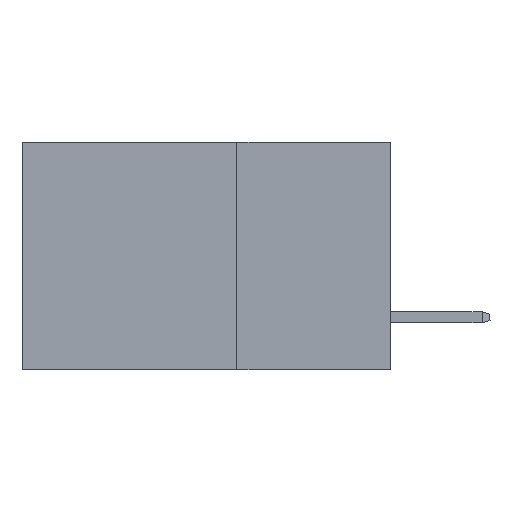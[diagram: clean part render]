
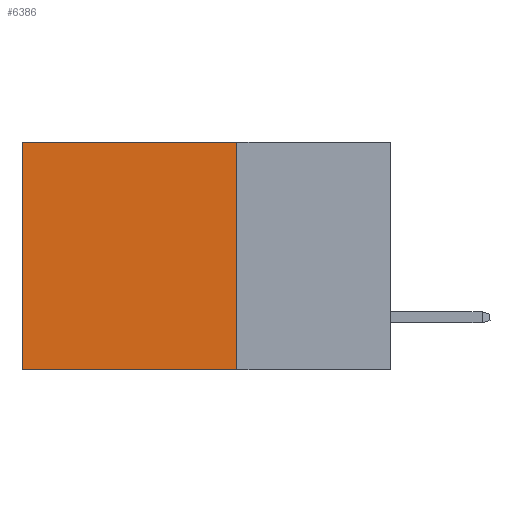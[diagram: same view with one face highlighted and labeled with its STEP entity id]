
A CAD part, left-side view. The second image highlights one B-rep face of the part: STEP entity #6386.
In plain terms, the highlighted planar face has unit normal (-1, 0, 0).
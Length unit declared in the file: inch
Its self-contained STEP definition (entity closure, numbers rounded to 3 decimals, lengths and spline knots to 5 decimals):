
#364 = CARTESIAN_POINT ( 'NONE',  ( 0.2875, 0.6, -0.37 ) ) ;
#1984 = CARTESIAN_POINT ( 'NONE',  ( 0.2875, 0.25, -0.37 ) ) ;
#2089 = DIRECTION ( 'NONE',  ( 0., 1., 0. ) ) ;
#3201 = EDGE_CURVE ( 'NONE', #13174, #11558, #13690, .T. ) ;
#3817 = ORIENTED_EDGE ( 'NONE', *, *, #20676, .F. ) ;
#4170 = ORIENTED_EDGE ( 'NONE', *, *, #3201, .T. ) ;
#4870 = CARTESIAN_POINT ( 'NONE',  ( 0.2875, 0.6, 0. ) ) ;
#5014 = VERTEX_POINT ( 'NONE', #11487 ) ;
#5525 = EDGE_CURVE ( 'NONE', #5014, #10387, #21760, .T. ) ;
#6386 = ADVANCED_FACE ( 'NONE', ( #8732 ), #9446, .F. ) ;
#7479 = CARTESIAN_POINT ( 'NONE',  ( 0.2875, 0.25, 0. ) ) ;
#8732 = FACE_OUTER_BOUND ( 'NONE', #17530, .T. ) ;
#9446 = PLANE ( 'NONE',  #27408 ) ;
#9730 = CARTESIAN_POINT ( 'NONE',  ( 0.2875, 0.25, 0. ) ) ;
#10387 = VERTEX_POINT ( 'NONE', #364 ) ;
#10723 = CARTESIAN_POINT ( 'NONE',  ( 0.2875, 0.6, 0. ) ) ;
#10885 = VECTOR ( 'NONE', #28116, 39.37008 ) ;
#11487 = CARTESIAN_POINT ( 'NONE',  ( 0.2875, 0.25, -0.37 ) ) ;
#11558 = VERTEX_POINT ( 'NONE', #4870 ) ;
#13174 = VERTEX_POINT ( 'NONE', #24351 ) ;
#13477 = LINE ( 'NONE', #9730, #25055 ) ;
#13690 = LINE ( 'NONE', #7479, #19503 ) ;
#13816 = DIRECTION ( 'NONE',  ( 0., 0., -1. ) ) ;
#14179 = EDGE_CURVE ( 'NONE', #11558, #10387, #28245, .T. ) ;
#17530 = EDGE_LOOP ( 'NONE', ( #19243, #17594, #3817, #4170 ) ) ;
#17594 = ORIENTED_EDGE ( 'NONE', *, *, #5525, .F. ) ;
#18402 = DIRECTION ( 'NONE',  ( 0., 0., -1. ) ) ;
#19243 = ORIENTED_EDGE ( 'NONE', *, *, #14179, .T. ) ;
#19503 = VECTOR ( 'NONE', #2089, 39.37008 ) ;
#20676 = EDGE_CURVE ( 'NONE', #13174, #5014, #13477, .T. ) ;
#21760 = LINE ( 'NONE', #1984, #26078 ) ;
#24351 = CARTESIAN_POINT ( 'NONE',  ( 0.2875, 0.25, 0. ) ) ;
#24649 = CARTESIAN_POINT ( 'NONE',  ( 0.2875, 0.25, 0. ) ) ;
#25055 = VECTOR ( 'NONE', #18402, 39.37008 ) ;
#26078 = VECTOR ( 'NONE', #28215, 39.37008 ) ;
#26808 = DIRECTION ( 'NONE',  ( 1., 0., 0. ) ) ;
#27408 = AXIS2_PLACEMENT_3D ( 'NONE', #24649, #26808, #13816 ) ;
#28116 = DIRECTION ( 'NONE',  ( 0., 0., -1. ) ) ;
#28215 = DIRECTION ( 'NONE',  ( 0., 1., 0. ) ) ;
#28245 = LINE ( 'NONE', #10723, #10885 ) ;
